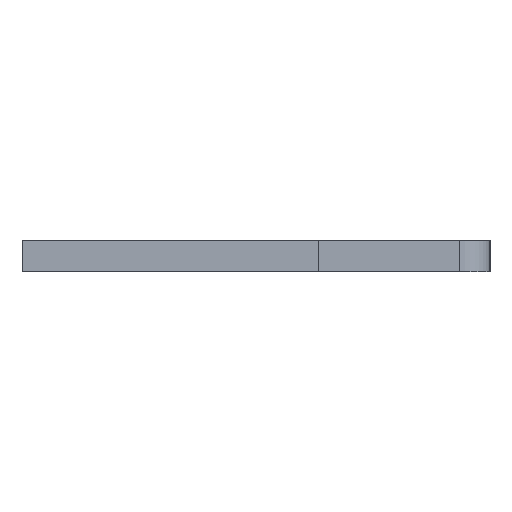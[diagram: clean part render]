
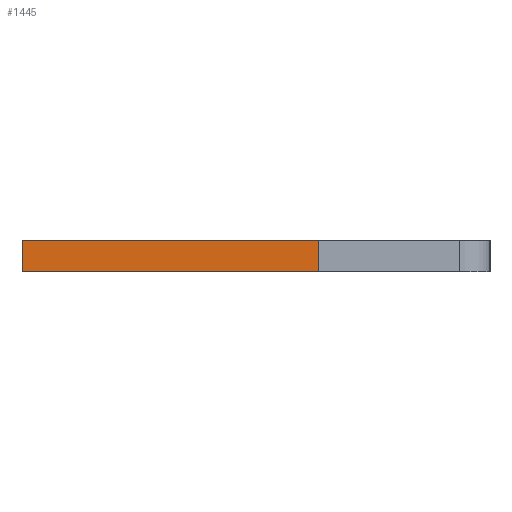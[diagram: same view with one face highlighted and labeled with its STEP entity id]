
A CAD part, left-side view. The second image highlights one B-rep face of the part: STEP entity #1445.
In plain terms, the highlighted face is planar.
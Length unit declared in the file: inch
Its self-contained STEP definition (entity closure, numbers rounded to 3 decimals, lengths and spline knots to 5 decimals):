
#41 = DIRECTION ( 'NONE',  ( -1., 0., 0. ) ) ;
#111 = VECTOR ( 'NONE', #41, 39.37008 ) ;
#198 = ORIENTED_EDGE ( 'NONE', *, *, #1756, .T. ) ;
#234 = LINE ( 'NONE', #1995, #1718 ) ;
#236 = DIRECTION ( 'NONE',  ( 0., 0., 1. ) ) ;
#282 = EDGE_LOOP ( 'NONE', ( #1126, #1493, #1322, #198 ) ) ;
#314 = VERTEX_POINT ( 'NONE', #2025 ) ;
#388 = CARTESIAN_POINT ( 'NONE',  ( -0.01, 0.15, -0.04 ) ) ;
#434 = CARTESIAN_POINT ( 'NONE',  ( -0.01, -0.04, -0.04 ) ) ;
#444 = CARTESIAN_POINT ( 'NONE',  ( 0.01, 0.15, -0.04 ) ) ;
#551 = DIRECTION ( 'NONE',  ( 0., 1., 0. ) ) ;
#593 = VERTEX_POINT ( 'NONE', #1125 ) ;
#741 = EDGE_CURVE ( 'NONE', #1339, #1213, #784, .T. ) ;
#784 = LINE ( 'NONE', #917, #1904 ) ;
#917 = CARTESIAN_POINT ( 'NONE',  ( -0.01, 0.15, -0.04 ) ) ;
#1024 = LINE ( 'NONE', #2158, #111 ) ;
#1034 = CARTESIAN_POINT ( 'NONE',  ( 0.01, 0.15, -0.04 ) ) ;
#1125 = CARTESIAN_POINT ( 'NONE',  ( 0.01, 0.15, -0.04 ) ) ;
#1126 = ORIENTED_EDGE ( 'NONE', *, *, #741, .T. ) ;
#1213 = VERTEX_POINT ( 'NONE', #388 ) ;
#1260 = VECTOR ( 'NONE', #1424, 39.37008 ) ;
#1262 = AXIS2_PLACEMENT_3D ( 'NONE', #444, #236, #1793 ) ;
#1322 = ORIENTED_EDGE ( 'NONE', *, *, #1526, .F. ) ;
#1339 = VERTEX_POINT ( 'NONE', #434 ) ;
#1409 = PLANE ( 'NONE',  #1262 ) ;
#1424 = DIRECTION ( 'NONE',  ( -1., 0., 0. ) ) ;
#1445 = ADVANCED_FACE ( 'NONE', ( #2397 ), #1409, .F. ) ;
#1453 = EDGE_CURVE ( 'NONE', #593, #1213, #2099, .T. ) ;
#1493 = ORIENTED_EDGE ( 'NONE', *, *, #1453, .F. ) ;
#1526 = EDGE_CURVE ( 'NONE', #314, #593, #234, .T. ) ;
#1718 = VECTOR ( 'NONE', #2167, 39.37008 ) ;
#1756 = EDGE_CURVE ( 'NONE', #314, #1339, #1024, .T. ) ;
#1793 = DIRECTION ( 'NONE',  ( 1., 0., 0. ) ) ;
#1904 = VECTOR ( 'NONE', #551, 39.37008 ) ;
#1995 = CARTESIAN_POINT ( 'NONE',  ( 0.01, 0.15, -0.04 ) ) ;
#2025 = CARTESIAN_POINT ( 'NONE',  ( 0.01, -0.04, -0.04 ) ) ;
#2099 = LINE ( 'NONE', #1034, #1260 ) ;
#2158 = CARTESIAN_POINT ( 'NONE',  ( 0.01, -0.04, -0.04 ) ) ;
#2167 = DIRECTION ( 'NONE',  ( 0., 1., 0. ) ) ;
#2397 = FACE_OUTER_BOUND ( 'NONE', #282, .T. ) ;
